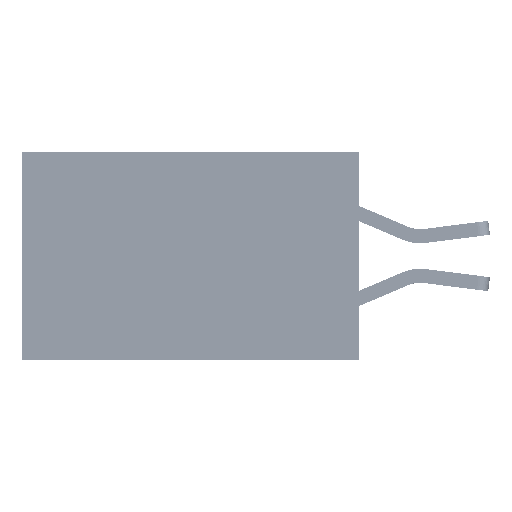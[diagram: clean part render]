
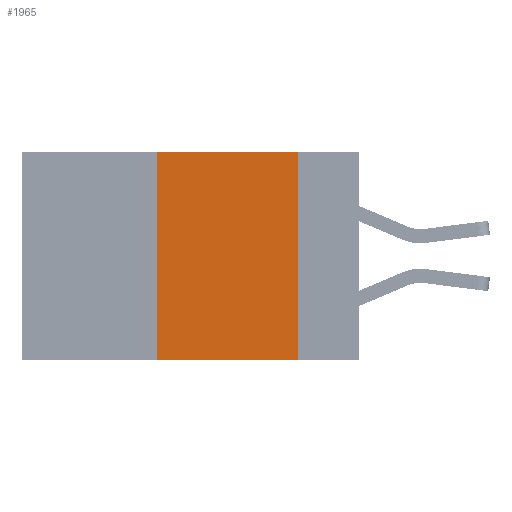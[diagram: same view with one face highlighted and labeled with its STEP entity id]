
A CAD part, left-side view. The second image highlights one B-rep face of the part: STEP entity #1965.
In plain terms, the highlighted planar face has unit normal (-1, 0, 0).
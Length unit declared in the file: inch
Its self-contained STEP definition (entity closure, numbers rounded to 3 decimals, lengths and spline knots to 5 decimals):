
#69 = DIRECTION ( 'NONE',  ( 0., 0., -1. ) ) ;
#80 = VERTEX_POINT ( 'NONE', #36645 ) ;
#1965 = ADVANCED_FACE ( 'NONE', ( #6017 ), #2335, .F. ) ;
#2335 = PLANE ( 'NONE',  #45330 ) ;
#3448 = ORIENTED_EDGE ( 'NONE', *, *, #26767, .T. ) ;
#4340 = DIRECTION ( 'NONE',  ( 0., -1., 0. ) ) ;
#6017 = FACE_OUTER_BOUND ( 'NONE', #28243, .T. ) ;
#7835 = CARTESIAN_POINT ( 'NONE',  ( 0., 0.6, 0. ) ) ;
#11379 = EDGE_CURVE ( 'NONE', #80, #29462, #12834, .T. ) ;
#12723 = VERTEX_POINT ( 'NONE', #27851 ) ;
#12834 = LINE ( 'NONE', #45005, #21612 ) ;
#14863 = DIRECTION ( 'NONE',  ( 0., -1., 0. ) ) ;
#15184 = VECTOR ( 'NONE', #14863, 39.37008 ) ;
#15602 = CARTESIAN_POINT ( 'NONE',  ( 0., 0.11, 0. ) ) ;
#16132 = VERTEX_POINT ( 'NONE', #15602 ) ;
#17538 = LINE ( 'NONE', #7835, #15184 ) ;
#17697 = LINE ( 'NONE', #22355, #26984 ) ;
#18968 = DIRECTION ( 'NONE',  ( 0., 0., 1. ) ) ;
#21612 = VECTOR ( 'NONE', #18968, 39.37008 ) ;
#22355 = CARTESIAN_POINT ( 'NONE',  ( 0., 0.11, 0. ) ) ;
#26767 = EDGE_CURVE ( 'NONE', #80, #12723, #44410, .T. ) ;
#26984 = VECTOR ( 'NONE', #69, 39.37008 ) ;
#27338 = EDGE_CURVE ( 'NONE', #29462, #16132, #17538, .T. ) ;
#27479 = VECTOR ( 'NONE', #4340, 39.37008 ) ;
#27851 = CARTESIAN_POINT ( 'NONE',  ( 0., 0.11, -0.37 ) ) ;
#28243 = EDGE_LOOP ( 'NONE', ( #37968, #44429, #38994, #3448 ) ) ;
#28518 = DIRECTION ( 'NONE',  ( 0., 0., -1. ) ) ;
#29462 = VERTEX_POINT ( 'NONE', #46365 ) ;
#36645 = CARTESIAN_POINT ( 'NONE',  ( 0., 0.36, -0.37 ) ) ;
#37907 = CARTESIAN_POINT ( 'NONE',  ( 0., 0.6, -0.37 ) ) ;
#37968 = ORIENTED_EDGE ( 'NONE', *, *, #45316, .F. ) ;
#38994 = ORIENTED_EDGE ( 'NONE', *, *, #11379, .F. ) ;
#43680 = DIRECTION ( 'NONE',  ( 1., 0., 0. ) ) ;
#44410 = LINE ( 'NONE', #37907, #27479 ) ;
#44429 = ORIENTED_EDGE ( 'NONE', *, *, #27338, .F. ) ;
#45005 = CARTESIAN_POINT ( 'NONE',  ( 0., 0.36, 0. ) ) ;
#45316 = EDGE_CURVE ( 'NONE', #16132, #12723, #17697, .T. ) ;
#45330 = AXIS2_PLACEMENT_3D ( 'NONE', #46937, #43680, #28518 ) ;
#46365 = CARTESIAN_POINT ( 'NONE',  ( 0., 0.36, 0. ) ) ;
#46937 = CARTESIAN_POINT ( 'NONE',  ( 0., 0.6, 0. ) ) ;
